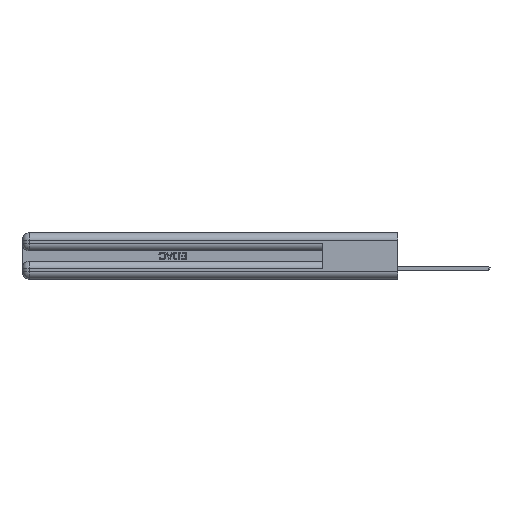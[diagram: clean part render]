
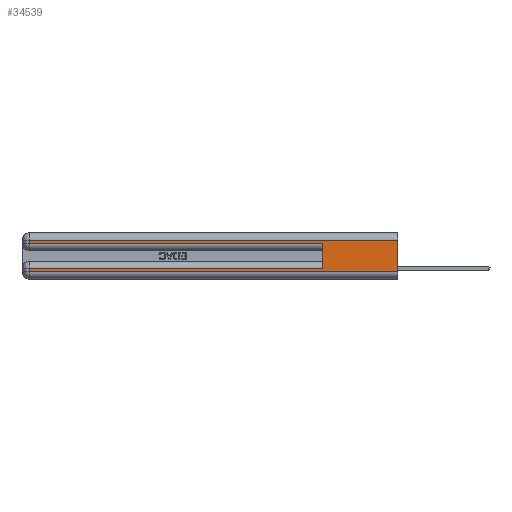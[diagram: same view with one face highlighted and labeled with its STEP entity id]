
A CAD part, left-side view. The second image highlights one B-rep face of the part: STEP entity #34539.
In plain terms, the highlighted planar face has unit normal (-1, 0, 0).
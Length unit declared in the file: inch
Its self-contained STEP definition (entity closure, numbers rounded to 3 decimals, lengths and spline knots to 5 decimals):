
#7 = EDGE_CURVE ( 'NONE', #25890, #9279, #35822, .T. ) ;
#331 = EDGE_CURVE ( 'NONE', #44004, #47805, #30238, .T. ) ;
#3964 = AXIS2_PLACEMENT_3D ( 'NONE', #24318, #16535, #24480 ) ;
#5049 = ORIENTED_EDGE ( 'NONE', *, *, #20227, .T. ) ;
#5384 = EDGE_CURVE ( 'NONE', #19410, #9279, #49437, .T. ) ;
#5415 = CARTESIAN_POINT ( 'NONE',  ( 0., 0., 0.06 ) ) ;
#6019 = CARTESIAN_POINT ( 'NONE',  ( 0., 2.94, 0.37 ) ) ;
#6870 = EDGE_CURVE ( 'NONE', #45764, #47805, #47340, .T. ) ;
#6966 = EDGE_CURVE ( 'NONE', #25890, #24471, #28604, .T. ) ;
#7948 = EDGE_CURVE ( 'NONE', #44004, #39518, #13012, .T. ) ;
#9279 = VERTEX_POINT ( 'NONE', #5415 ) ;
#10253 = CARTESIAN_POINT ( 'NONE',  ( 0., 0., 0.37 ) ) ;
#10881 = ORIENTED_EDGE ( 'NONE', *, *, #7948, .T. ) ;
#11710 = CARTESIAN_POINT ( 'NONE',  ( 0., 2.94, 0.31 ) ) ;
#11929 = VECTOR ( 'NONE', #41537, 39.37008 ) ;
#12623 = ORIENTED_EDGE ( 'NONE', *, *, #6966, .T. ) ;
#13012 = LINE ( 'NONE', #31081, #42193 ) ;
#13561 = DIRECTION ( 'NONE',  ( 0., 0., -1. ) ) ;
#16033 = PLANE ( 'NONE',  #3964 ) ;
#16535 = DIRECTION ( 'NONE',  ( 1., 0., 0. ) ) ;
#18963 = DIRECTION ( 'NONE',  ( 0., 0., 1. ) ) ;
#19025 = ORIENTED_EDGE ( 'NONE', *, *, #331, .F. ) ;
#19410 = VERTEX_POINT ( 'NONE', #22517 ) ;
#20227 = EDGE_CURVE ( 'NONE', #24471, #45764, #43585, .T. ) ;
#21140 = LINE ( 'NONE', #41654, #26774 ) ;
#22517 = CARTESIAN_POINT ( 'NONE',  ( 0., 2.94, 0.06 ) ) ;
#22646 = ORIENTED_EDGE ( 'NONE', *, *, #5384, .T. ) ;
#23096 = VECTOR ( 'NONE', #26671, 39.37008 ) ;
#24032 = VECTOR ( 'NONE', #49328, 39.37008 ) ;
#24265 = EDGE_CURVE ( 'NONE', #39518, #19410, #21140, .T. ) ;
#24318 = CARTESIAN_POINT ( 'NONE',  ( 0., 0., 0.37 ) ) ;
#24471 = VERTEX_POINT ( 'NONE', #11710 ) ;
#24480 = DIRECTION ( 'NONE',  ( 0., 0., -1. ) ) ;
#25890 = VERTEX_POINT ( 'NONE', #44613 ) ;
#26671 = DIRECTION ( 'NONE',  ( 0., 1., 0. ) ) ;
#26774 = VECTOR ( 'NONE', #13561, 39.37008 ) ;
#27578 = CARTESIAN_POINT ( 'NONE',  ( 0., 0.6, 0.085 ) ) ;
#28604 = LINE ( 'NONE', #42112, #23096 ) ;
#30238 = LINE ( 'NONE', #38740, #35775 ) ;
#31081 = CARTESIAN_POINT ( 'NONE',  ( 0., 0., 0.085 ) ) ;
#31502 = CARTESIAN_POINT ( 'NONE',  ( 0., 2.94, 0.085 ) ) ;
#32637 = EDGE_LOOP ( 'NONE', ( #39160, #12623, #5049, #41866, #19025, #10881, #42894, #22646 ) ) ;
#34539 = ADVANCED_FACE ( 'NONE', ( #42117 ), #16033, .F. ) ;
#35775 = VECTOR ( 'NONE', #18963, 39.37008 ) ;
#35822 = LINE ( 'NONE', #10253, #24032 ) ;
#37942 = VECTOR ( 'NONE', #42696, 39.37008 ) ;
#38175 = CARTESIAN_POINT ( 'NONE',  ( 0., 0., 0.285 ) ) ;
#38627 = CARTESIAN_POINT ( 'NONE',  ( 0., 0.6, 0.285 ) ) ;
#38740 = CARTESIAN_POINT ( 'NONE',  ( 0., 0.6, 0.145 ) ) ;
#39160 = ORIENTED_EDGE ( 'NONE', *, *, #7, .F. ) ;
#39518 = VERTEX_POINT ( 'NONE', #31502 ) ;
#41537 = DIRECTION ( 'NONE',  ( 0., 0., -1. ) ) ;
#41654 = CARTESIAN_POINT ( 'NONE',  ( 0., 2.94, 0.37 ) ) ;
#41866 = ORIENTED_EDGE ( 'NONE', *, *, #6870, .T. ) ;
#41901 = VECTOR ( 'NONE', #46047, 39.37008 ) ;
#42112 = CARTESIAN_POINT ( 'NONE',  ( 0., 0., 0.31 ) ) ;
#42117 = FACE_OUTER_BOUND ( 'NONE', #32637, .T. ) ;
#42193 = VECTOR ( 'NONE', #42942, 39.37008 ) ;
#42696 = DIRECTION ( 'NONE',  ( 0., -1., 0. ) ) ;
#42894 = ORIENTED_EDGE ( 'NONE', *, *, #24265, .T. ) ;
#42942 = DIRECTION ( 'NONE',  ( 0., 1., 0. ) ) ;
#43065 = CARTESIAN_POINT ( 'NONE',  ( 0., 2.94, 0.285 ) ) ;
#43585 = LINE ( 'NONE', #6019, #11929 ) ;
#44004 = VERTEX_POINT ( 'NONE', #27578 ) ;
#44613 = CARTESIAN_POINT ( 'NONE',  ( 0., 0., 0.31 ) ) ;
#44638 = CARTESIAN_POINT ( 'NONE',  ( 0., 0., 0.06 ) ) ;
#45764 = VERTEX_POINT ( 'NONE', #43065 ) ;
#46047 = DIRECTION ( 'NONE',  ( 0., -1., 0. ) ) ;
#47340 = LINE ( 'NONE', #38175, #37942 ) ;
#47805 = VERTEX_POINT ( 'NONE', #38627 ) ;
#49328 = DIRECTION ( 'NONE',  ( 0., 0., -1. ) ) ;
#49437 = LINE ( 'NONE', #44638, #41901 ) ;
